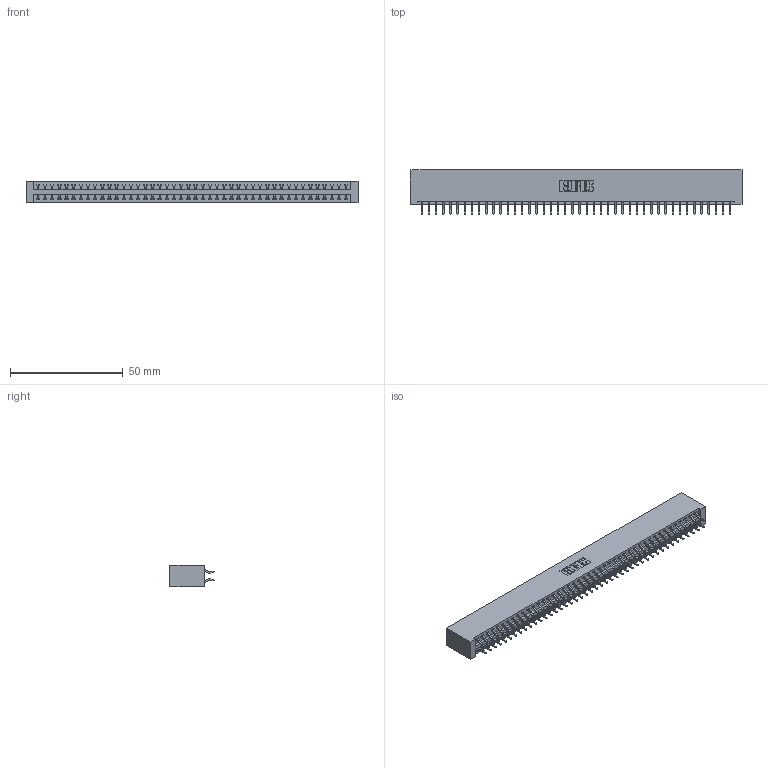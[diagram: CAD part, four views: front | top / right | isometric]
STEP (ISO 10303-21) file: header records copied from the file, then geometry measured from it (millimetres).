
FILE_DESCRIPTION (( 'STEP AP203' ), '1' );
FILE_NAME ('346-088-556-201.STEP', '2018-08-30T00:36:49', ( '' ), ( '' ), 'SwSTEP 2.0', 'SolidWorks 2016', '' );
FILE_SCHEMA (( 'CONFIG_CONTROL_DESIGN' ));
Length unit declared in the file: inch
Products named in the file (3): 346 Part_No Mounting Lugs; 345-292-001_556 Tail; 346-088-556-201
Assembly tree (89 placements, depth 2):
  346-088-556-201
    346 Part_No Mounting Lugs
    345-292-001_556 Tail  x88
Bounding box: 146.94 x 19.57 x 9.4 mm (x, y, z)
Volume: 14913.7 mm3; surface area: 20612.8 mm2
Topology: 89 solids, 89 shells, 5218 faces, 15529 edges, 10234 vertices
Faces by surface type: plane 3504, cylinder 1714
Entity records: 28389 total; most frequent: CARTESIAN_POINT 4688, ORIENTED_EDGE 4610, DIRECTION 4165, EDGE_CURVE 2305, LINE 1997, VECTOR 1997, VERTEX_POINT 1534, AXIS2_PLACEMENT_3D 1084
